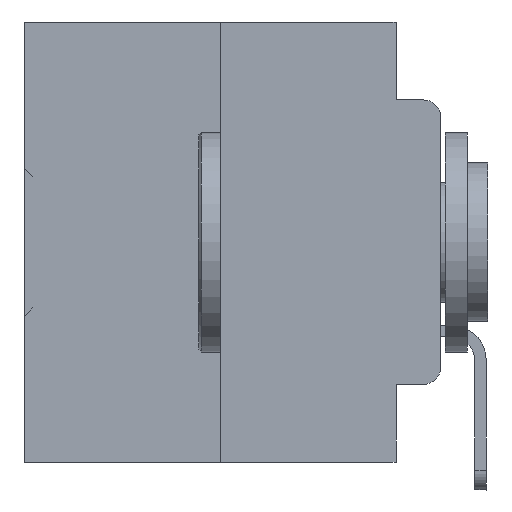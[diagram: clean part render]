
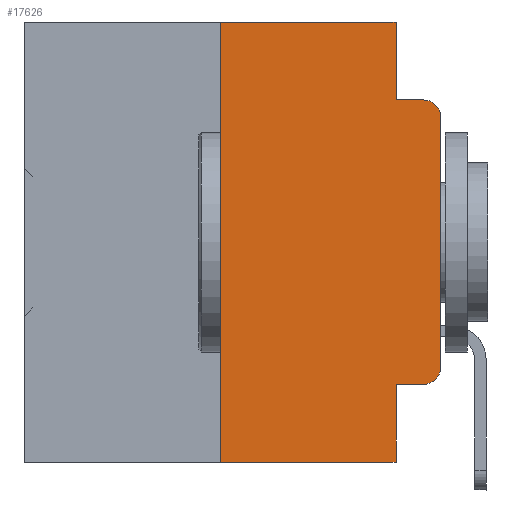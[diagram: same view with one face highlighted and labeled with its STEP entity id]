
A CAD part, left-side view. The second image highlights one B-rep face of the part: STEP entity #17626.
In plain terms, the highlighted planar face has unit normal (-1, 0, 0).
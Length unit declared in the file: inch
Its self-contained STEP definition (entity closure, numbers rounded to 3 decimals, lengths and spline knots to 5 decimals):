
#102 = EDGE_CURVE ( 'NONE', #1635, #13770, #25163, .T. ) ;
#321 = ORIENTED_EDGE ( 'NONE', *, *, #5844, .F. ) ;
#1273 = DIRECTION ( 'NONE',  ( 0., 0., 1. ) ) ;
#1364 = ORIENTED_EDGE ( 'NONE', *, *, #10084, .T. ) ;
#1465 = VECTOR ( 'NONE', #1273, 39.37008 ) ;
#1635 = VERTEX_POINT ( 'NONE', #35982 ) ;
#1739 = EDGE_CURVE ( 'NONE', #17782, #35069, #34298, .T. ) ;
#1920 = DIRECTION ( 'NONE',  ( 0., 0., -1. ) ) ;
#2110 = DIRECTION ( 'NONE',  ( 0., -1., 0. ) ) ;
#2843 = PLANE ( 'NONE',  #17062 ) ;
#3235 = VERTEX_POINT ( 'NONE', #26410 ) ;
#3317 = EDGE_LOOP ( 'NONE', ( #12602, #1364, #30333, #16708, #29971, #321, #14566, #31861, #7267, #10706 ) ) ;
#4096 = EDGE_CURVE ( 'NONE', #3235, #1635, #20888, .T. ) ;
#5078 = CARTESIAN_POINT ( 'NONE',  ( 0., 0.25, 0. ) ) ;
#5265 = LINE ( 'NONE', #37763, #7563 ) ;
#5376 = DIRECTION ( 'NONE',  ( 0., 0., -1. ) ) ;
#5685 = DIRECTION ( 'NONE',  ( 0., 0., -1. ) ) ;
#5725 = VERTEX_POINT ( 'NONE', #6221 ) ;
#5844 = EDGE_CURVE ( 'NONE', #26436, #17782, #13444, .T. ) ;
#6221 = CARTESIAN_POINT ( 'NONE',  ( 0., 0.02, -0.0885 ) ) ;
#6718 = CARTESIAN_POINT ( 'NONE',  ( 0., 0.473, 0. ) ) ;
#6787 = DIRECTION ( 'NONE',  ( 0., -1., 0. ) ) ;
#7267 = ORIENTED_EDGE ( 'NONE', *, *, #4096, .T. ) ;
#7563 = VECTOR ( 'NONE', #5685, 39.37008 ) ;
#9516 = DIRECTION ( 'NONE',  ( 0., 0., 1. ) ) ;
#10016 = CARTESIAN_POINT ( 'NONE',  ( 0., 0.051, -0.4115 ) ) ;
#10035 = EDGE_CURVE ( 'NONE', #35069, #33590, #16354, .T. ) ;
#10084 = EDGE_CURVE ( 'NONE', #11957, #5725, #23269, .T. ) ;
#10706 = ORIENTED_EDGE ( 'NONE', *, *, #102, .T. ) ;
#10780 = CARTESIAN_POINT ( 'NONE',  ( 0., 0., -0.3915 ) ) ;
#11957 = VERTEX_POINT ( 'NONE', #27196 ) ;
#12587 = DIRECTION ( 'NONE',  ( 0., -1., 0. ) ) ;
#12602 = ORIENTED_EDGE ( 'NONE', *, *, #19885, .T. ) ;
#12701 = DIRECTION ( 'NONE',  ( 0., -1., 0. ) ) ;
#13444 = LINE ( 'NONE', #26795, #19404 ) ;
#13715 = VECTOR ( 'NONE', #12587, 39.37008 ) ;
#13770 = VERTEX_POINT ( 'NONE', #10780 ) ;
#14355 = EDGE_CURVE ( 'NONE', #3235, #36434, #5265, .T. ) ;
#14458 = DIRECTION ( 'NONE',  ( -1., 0., 0. ) ) ;
#14566 = ORIENTED_EDGE ( 'NONE', *, *, #22647, .T. ) ;
#16354 = LINE ( 'NONE', #21626, #26425 ) ;
#16708 = ORIENTED_EDGE ( 'NONE', *, *, #10035, .F. ) ;
#17062 = AXIS2_PLACEMENT_3D ( 'NONE', #21750, #33865, #5376 ) ;
#17626 = ADVANCED_FACE ( 'NONE', ( #25590 ), #2843, .F. ) ;
#17686 = CARTESIAN_POINT ( 'NONE',  ( 0., 0.02, -0.3915 ) ) ;
#17782 = VERTEX_POINT ( 'NONE', #5078 ) ;
#18138 = CARTESIAN_POINT ( 'NONE',  ( 0., 0.051, -0.5 ) ) ;
#19404 = VECTOR ( 'NONE', #9516, 39.37008 ) ;
#19885 = EDGE_CURVE ( 'NONE', #13770, #11957, #26653, .T. ) ;
#20426 = DIRECTION ( 'NONE',  ( 0., 0., -1. ) ) ;
#20652 = DIRECTION ( 'NONE',  ( -1., 0., 0. ) ) ;
#20888 = LINE ( 'NONE', #10016, #35062 ) ;
#21626 = CARTESIAN_POINT ( 'NONE',  ( 0., 0.051, 0. ) ) ;
#21750 = CARTESIAN_POINT ( 'NONE',  ( 0., 0.473, 0. ) ) ;
#22647 = EDGE_CURVE ( 'NONE', #26436, #36434, #35575, .T. ) ;
#23269 = CIRCLE ( 'NONE', #26176, 0.02 ) ;
#25107 = VECTOR ( 'NONE', #6787, 39.37008 ) ;
#25163 = CIRCLE ( 'NONE', #26190, 0.02 ) ;
#25590 = FACE_OUTER_BOUND ( 'NONE', #3317, .T. ) ;
#26176 = AXIS2_PLACEMENT_3D ( 'NONE', #32099, #14458, #37619 ) ;
#26190 = AXIS2_PLACEMENT_3D ( 'NONE', #17686, #20652, #20426 ) ;
#26410 = CARTESIAN_POINT ( 'NONE',  ( 0., 0.051, -0.4115 ) ) ;
#26425 = VECTOR ( 'NONE', #1920, 39.37008 ) ;
#26436 = VERTEX_POINT ( 'NONE', #28158 ) ;
#26653 = LINE ( 'NONE', #33358, #1465 ) ;
#26795 = CARTESIAN_POINT ( 'NONE',  ( 0., 0.25, 0. ) ) ;
#27196 = CARTESIAN_POINT ( 'NONE',  ( 0., 0., -0.1085 ) ) ;
#28158 = CARTESIAN_POINT ( 'NONE',  ( 0., 0.25, -0.5 ) ) ;
#28902 = CARTESIAN_POINT ( 'NONE',  ( 0., 0.473, -0.5 ) ) ;
#29057 = CARTESIAN_POINT ( 'NONE',  ( 0., 0.051, 0. ) ) ;
#29971 = ORIENTED_EDGE ( 'NONE', *, *, #1739, .F. ) ;
#30333 = ORIENTED_EDGE ( 'NONE', *, *, #37120, .F. ) ;
#30891 = CARTESIAN_POINT ( 'NONE',  ( 0., 0.051, -0.0885 ) ) ;
#31056 = VECTOR ( 'NONE', #2110, 39.37008 ) ;
#31861 = ORIENTED_EDGE ( 'NONE', *, *, #14355, .F. ) ;
#32099 = CARTESIAN_POINT ( 'NONE',  ( 0., 0.02, -0.1085 ) ) ;
#32834 = LINE ( 'NONE', #30891, #31056 ) ;
#33358 = CARTESIAN_POINT ( 'NONE',  ( 0., 0., 0. ) ) ;
#33590 = VERTEX_POINT ( 'NONE', #34772 ) ;
#33865 = DIRECTION ( 'NONE',  ( 1., 0., 0. ) ) ;
#34298 = LINE ( 'NONE', #6718, #13715 ) ;
#34772 = CARTESIAN_POINT ( 'NONE',  ( 0., 0.051, -0.0885 ) ) ;
#35062 = VECTOR ( 'NONE', #12701, 39.37008 ) ;
#35069 = VERTEX_POINT ( 'NONE', #29057 ) ;
#35575 = LINE ( 'NONE', #28902, #25107 ) ;
#35982 = CARTESIAN_POINT ( 'NONE',  ( 0., 0.02, -0.4115 ) ) ;
#36434 = VERTEX_POINT ( 'NONE', #18138 ) ;
#37120 = EDGE_CURVE ( 'NONE', #33590, #5725, #32834, .T. ) ;
#37619 = DIRECTION ( 'NONE',  ( 0., 0., -1. ) ) ;
#37763 = CARTESIAN_POINT ( 'NONE',  ( 0., 0.051, 0. ) ) ;
